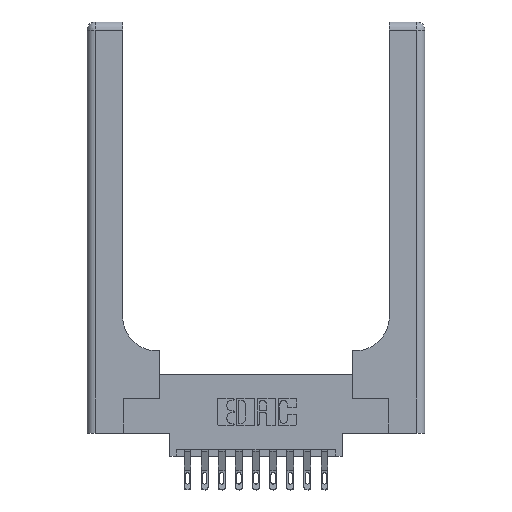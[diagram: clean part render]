
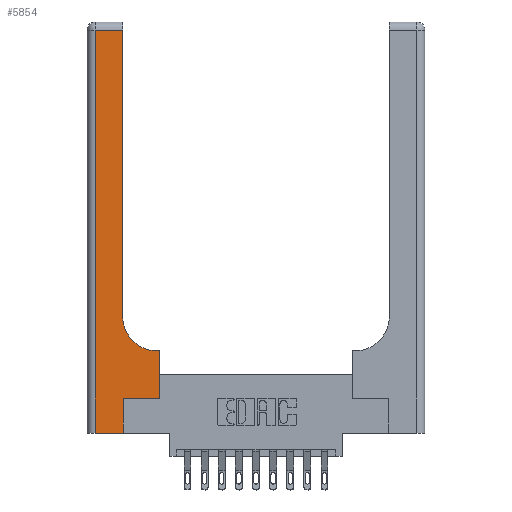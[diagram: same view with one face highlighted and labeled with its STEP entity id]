
A CAD part, top view. The second image highlights one B-rep face of the part: STEP entity #5854.
In plain terms, the highlighted planar face has unit normal (0, 0, 1).
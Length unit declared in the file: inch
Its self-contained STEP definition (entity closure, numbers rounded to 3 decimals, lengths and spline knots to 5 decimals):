
#66 = VERTEX_POINT ( 'NONE', #5166 ) ;
#105 = VERTEX_POINT ( 'NONE', #504 ) ;
#173 = ORIENTED_EDGE ( 'NONE', *, *, #5604, .T. ) ;
#348 = ORIENTED_EDGE ( 'NONE', *, *, #10677, .T. ) ;
#504 = CARTESIAN_POINT ( 'NONE',  ( 0.265, 0.25, 0.37 ) ) ;
#588 = LINE ( 'NONE', #5411, #14189 ) ;
#1087 = LINE ( 'NONE', #13794, #3879 ) ;
#1223 = VECTOR ( 'NONE', #5120, 39.37008 ) ;
#1376 = CARTESIAN_POINT ( 'NONE',  ( 0., 0., 0.37 ) ) ;
#1486 = AXIS2_PLACEMENT_3D ( 'NONE', #15521, #4013, #11522 ) ;
#1518 = DIRECTION ( 'NONE',  ( 1., 0., 0. ) ) ;
#1674 = ORIENTED_EDGE ( 'NONE', *, *, #6625, .T. ) ;
#2929 = ORIENTED_EDGE ( 'NONE', *, *, #13430, .T. ) ;
#3433 = LINE ( 'NONE', #13543, #4696 ) ;
#3745 = ORIENTED_EDGE ( 'NONE', *, *, #11535, .T. ) ;
#3879 = VECTOR ( 'NONE', #9956, 39.37008 ) ;
#4013 = DIRECTION ( 'NONE',  ( 0., 0., -1. ) ) ;
#4179 = ORIENTED_EDGE ( 'NONE', *, *, #13166, .T. ) ;
#4254 = DIRECTION ( 'NONE',  ( -1., 0., 0. ) ) ;
#4261 = LINE ( 'NONE', #7914, #6809 ) ;
#4484 = VERTEX_POINT ( 'NONE', #11121 ) ;
#4573 = EDGE_CURVE ( 'NONE', #10819, #4484, #1087, .T. ) ;
#4696 = VECTOR ( 'NONE', #7244, 39.37008 ) ;
#4947 = EDGE_LOOP ( 'NONE', ( #9367, #348, #4179, #3745, #10533, #8864, #1674, #173, #2929 ) ) ;
#5120 = DIRECTION ( 'NONE',  ( 0., 1., 0. ) ) ;
#5166 = CARTESIAN_POINT ( 'NONE',  ( 0.265, 0., 0.37 ) ) ;
#5411 = CARTESIAN_POINT ( 'NONE',  ( 0.06, 3., 0.37 ) ) ;
#5604 = EDGE_CURVE ( 'NONE', #8324, #16251, #3433, .T. ) ;
#5854 = ADVANCED_FACE ( 'NONE', ( #6815 ), #11763, .F. ) ;
#6524 = CIRCLE ( 'NONE', #1486, 0.25 ) ;
#6625 = EDGE_CURVE ( 'NONE', #7342, #8324, #9035, .T. ) ;
#6809 = VECTOR ( 'NONE', #9240, 39.37008 ) ;
#6815 = FACE_OUTER_BOUND ( 'NONE', #4947, .T. ) ;
#6951 = CARTESIAN_POINT ( 'NONE',  ( 0.51, 0.6, 0.37 ) ) ;
#7244 = DIRECTION ( 'NONE',  ( -1., 0., 0. ) ) ;
#7342 = VERTEX_POINT ( 'NONE', #9488 ) ;
#7700 = DIRECTION ( 'NONE',  ( 1., 0., 0. ) ) ;
#7900 = CARTESIAN_POINT ( 'NONE',  ( 0.26, 0.85, 0.37 ) ) ;
#7914 = CARTESIAN_POINT ( 'NONE',  ( 0.265, 0., 0.37 ) ) ;
#7931 = VERTEX_POINT ( 'NONE', #13159 ) ;
#8150 = CARTESIAN_POINT ( 'NONE',  ( 0., 3., 0.37 ) ) ;
#8324 = VERTEX_POINT ( 'NONE', #11713 ) ;
#8864 = ORIENTED_EDGE ( 'NONE', *, *, #9951, .T. ) ;
#9035 = LINE ( 'NONE', #9105, #1223 ) ;
#9105 = CARTESIAN_POINT ( 'NONE',  ( 0.528, 0.25, 0.37 ) ) ;
#9240 = DIRECTION ( 'NONE',  ( 0., 1., 0. ) ) ;
#9367 = ORIENTED_EDGE ( 'NONE', *, *, #4573, .T. ) ;
#9410 = CARTESIAN_POINT ( 'NONE',  ( 0., 2.94, 0.37 ) ) ;
#9488 = CARTESIAN_POINT ( 'NONE',  ( 0.528, 0.25, 0.37 ) ) ;
#9951 = EDGE_CURVE ( 'NONE', #105, #7342, #14200, .T. ) ;
#9956 = DIRECTION ( 'NONE',  ( 0., 1., 0. ) ) ;
#10454 = VECTOR ( 'NONE', #11972, 39.37008 ) ;
#10533 = ORIENTED_EDGE ( 'NONE', *, *, #14102, .T. ) ;
#10677 = EDGE_CURVE ( 'NONE', #4484, #7931, #11273, .T. ) ;
#10819 = VERTEX_POINT ( 'NONE', #7900 ) ;
#10867 = CARTESIAN_POINT ( 'NONE',  ( 0.06, 0., 0.37 ) ) ;
#11036 = DIRECTION ( 'NONE',  ( 0., -1., 0. ) ) ;
#11121 = CARTESIAN_POINT ( 'NONE',  ( 0.26, 2.94, 0.37 ) ) ;
#11160 = LINE ( 'NONE', #1376, #11791 ) ;
#11273 = LINE ( 'NONE', #9410, #10454 ) ;
#11522 = DIRECTION ( 'NONE',  ( 1., 0., 0. ) ) ;
#11535 = EDGE_CURVE ( 'NONE', #12016, #66, #11160, .T. ) ;
#11713 = CARTESIAN_POINT ( 'NONE',  ( 0.528, 0.6, 0.37 ) ) ;
#11763 = PLANE ( 'NONE',  #11792 ) ;
#11791 = VECTOR ( 'NONE', #7700, 39.37008 ) ;
#11792 = AXIS2_PLACEMENT_3D ( 'NONE', #8150, #15606, #4254 ) ;
#11943 = CARTESIAN_POINT ( 'NONE',  ( 0.265, 0.25, 0.37 ) ) ;
#11972 = DIRECTION ( 'NONE',  ( -1., 0., 0. ) ) ;
#12016 = VERTEX_POINT ( 'NONE', #10867 ) ;
#13159 = CARTESIAN_POINT ( 'NONE',  ( 0.06, 2.94, 0.37 ) ) ;
#13166 = EDGE_CURVE ( 'NONE', #7931, #12016, #588, .T. ) ;
#13430 = EDGE_CURVE ( 'NONE', #16251, #10819, #6524, .T. ) ;
#13543 = CARTESIAN_POINT ( 'NONE',  ( 0.26, 0.6, 0.37 ) ) ;
#13794 = CARTESIAN_POINT ( 'NONE',  ( 0.26, 3., 0.37 ) ) ;
#14102 = EDGE_CURVE ( 'NONE', #66, #105, #4261, .T. ) ;
#14189 = VECTOR ( 'NONE', #11036, 39.37008 ) ;
#14200 = LINE ( 'NONE', #11943, #15090 ) ;
#15090 = VECTOR ( 'NONE', #1518, 39.37008 ) ;
#15521 = CARTESIAN_POINT ( 'NONE',  ( 0.51, 0.85, 0.37 ) ) ;
#15606 = DIRECTION ( 'NONE',  ( 0., 0., -1. ) ) ;
#16251 = VERTEX_POINT ( 'NONE', #6951 ) ;
